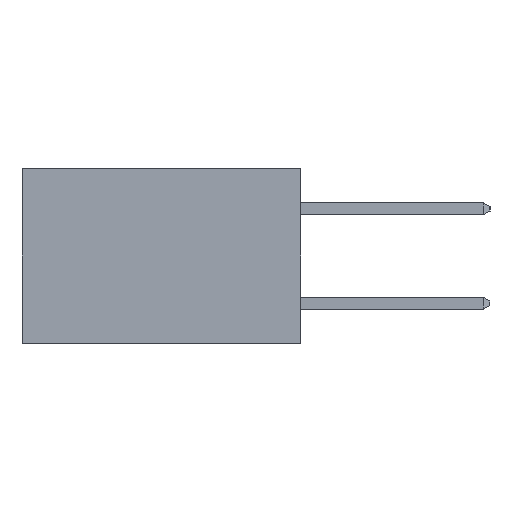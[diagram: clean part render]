
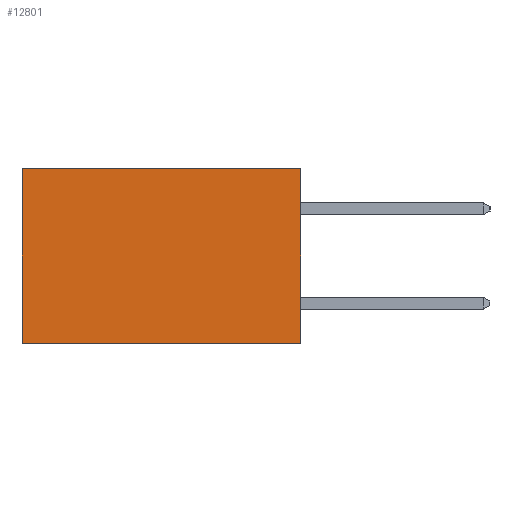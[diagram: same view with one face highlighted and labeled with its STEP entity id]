
A CAD part, left-side view. The second image highlights one B-rep face of the part: STEP entity #12801.
In plain terms, the highlighted planar face has unit normal (-1, 0, 0).
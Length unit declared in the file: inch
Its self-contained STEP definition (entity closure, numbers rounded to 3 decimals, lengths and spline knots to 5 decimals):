
#754 = ORIENTED_EDGE ( 'NONE', *, *, #6795, .F. ) ;
#1124 = FACE_OUTER_BOUND ( 'NONE', #4317, .T. ) ;
#1352 = LINE ( 'NONE', #6686, #8621 ) ;
#2950 = LINE ( 'NONE', #8837, #14239 ) ;
#3067 = CARTESIAN_POINT ( 'NONE',  ( 0.277, 0.59, -0.37 ) ) ;
#3310 = DIRECTION ( 'NONE',  ( 0., 0., -1. ) ) ;
#3410 = AXIS2_PLACEMENT_3D ( 'NONE', #7563, #11801, #3310 ) ;
#3497 = VERTEX_POINT ( 'NONE', #13215 ) ;
#4087 = DIRECTION ( 'NONE',  ( 0., 0., -1. ) ) ;
#4203 = CARTESIAN_POINT ( 'NONE',  ( 0.277, 0.59, 0. ) ) ;
#4264 = ORIENTED_EDGE ( 'NONE', *, *, #10827, .F. ) ;
#4317 = EDGE_LOOP ( 'NONE', ( #7607, #4264, #754, #15984 ) ) ;
#4344 = DIRECTION ( 'NONE',  ( 0., 1., 0. ) ) ;
#5949 = EDGE_CURVE ( 'NONE', #11450, #16071, #1352, .T. ) ;
#6581 = DIRECTION ( 'NONE',  ( 0., 0., -1. ) ) ;
#6686 = CARTESIAN_POINT ( 'NONE',  ( 0.277, 0.59, -0.37 ) ) ;
#6795 = EDGE_CURVE ( 'NONE', #3497, #15951, #10346, .T. ) ;
#7563 = CARTESIAN_POINT ( 'NONE',  ( 0.277, 0., -0.37 ) ) ;
#7607 = ORIENTED_EDGE ( 'NONE', *, *, #5949, .T. ) ;
#8517 = CARTESIAN_POINT ( 'NONE',  ( 0.277, 0., -0.37 ) ) ;
#8621 = VECTOR ( 'NONE', #6581, 39.37008 ) ;
#8837 = CARTESIAN_POINT ( 'NONE',  ( 0.277, 0., 0. ) ) ;
#8989 = EDGE_CURVE ( 'NONE', #3497, #11450, #2950, .T. ) ;
#9695 = CARTESIAN_POINT ( 'NONE',  ( 0.277, 0., -0.37 ) ) ;
#9984 = CARTESIAN_POINT ( 'NONE',  ( 0.277, 0., -0.37 ) ) ;
#10237 = DIRECTION ( 'NONE',  ( 0., 1., 0. ) ) ;
#10346 = LINE ( 'NONE', #9695, #16916 ) ;
#10402 = PLANE ( 'NONE',  #3410 ) ;
#10827 = EDGE_CURVE ( 'NONE', #15951, #16071, #13986, .T. ) ;
#11450 = VERTEX_POINT ( 'NONE', #4203 ) ;
#11801 = DIRECTION ( 'NONE',  ( 1., 0., 0. ) ) ;
#12801 = ADVANCED_FACE ( 'NONE', ( #1124 ), #10402, .F. ) ;
#13215 = CARTESIAN_POINT ( 'NONE',  ( 0.277, 0., 0. ) ) ;
#13540 = VECTOR ( 'NONE', #4344, 39.37008 ) ;
#13986 = LINE ( 'NONE', #9984, #13540 ) ;
#14239 = VECTOR ( 'NONE', #10237, 39.37008 ) ;
#15951 = VERTEX_POINT ( 'NONE', #8517 ) ;
#15984 = ORIENTED_EDGE ( 'NONE', *, *, #8989, .T. ) ;
#16071 = VERTEX_POINT ( 'NONE', #3067 ) ;
#16916 = VECTOR ( 'NONE', #4087, 39.37008 ) ;
